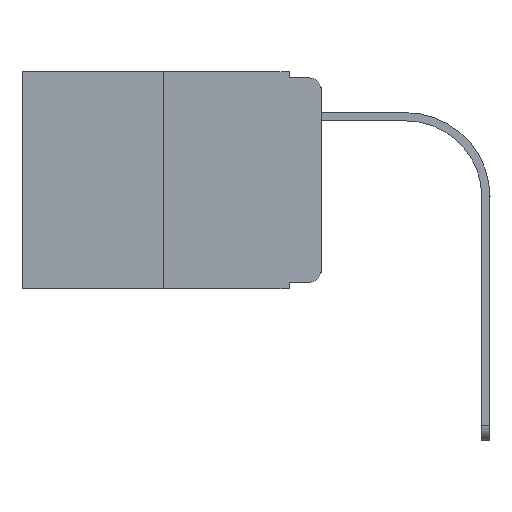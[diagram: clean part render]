
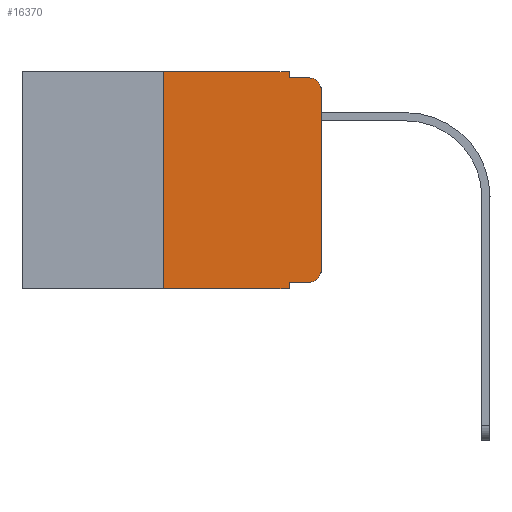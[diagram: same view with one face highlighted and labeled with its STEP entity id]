
A CAD part, left-side view. The second image highlights one B-rep face of the part: STEP entity #16370.
In plain terms, the highlighted planar face has unit normal (-1, 0, 0).
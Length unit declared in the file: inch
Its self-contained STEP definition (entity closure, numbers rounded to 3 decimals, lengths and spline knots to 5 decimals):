
#97 = DIRECTION ( 'NONE',  ( 0., -1., 0. ) ) ;
#289 = CARTESIAN_POINT ( 'NONE',  ( 0., 0.051, -0.333 ) ) ;
#323 = LINE ( 'NONE', #18625, #15803 ) ;
#576 = VERTEX_POINT ( 'NONE', #289 ) ;
#582 = DIRECTION ( 'NONE',  ( 0., 0., -1. ) ) ;
#863 = CARTESIAN_POINT ( 'NONE',  ( 0., 0., -0.03 ) ) ;
#1240 = ORIENTED_EDGE ( 'NONE', *, *, #13371, .F. ) ;
#1433 = EDGE_CURVE ( 'NONE', #3474, #18431, #18439, .T. ) ;
#1814 = CARTESIAN_POINT ( 'NONE',  ( 0., 0.473, 0. ) ) ;
#1886 = LINE ( 'NONE', #16724, #15252 ) ;
#2597 = LINE ( 'NONE', #4311, #8009 ) ;
#2624 = CARTESIAN_POINT ( 'NONE',  ( 0., 0.051, -0.01 ) ) ;
#2825 = VERTEX_POINT ( 'NONE', #2624 ) ;
#3166 = EDGE_CURVE ( 'NONE', #12573, #2825, #2597, .T. ) ;
#3474 = VERTEX_POINT ( 'NONE', #19797 ) ;
#3477 = CARTESIAN_POINT ( 'NONE',  ( 0., 0.25, -0.343 ) ) ;
#3517 = ORIENTED_EDGE ( 'NONE', *, *, #7996, .T. ) ;
#3905 = EDGE_CURVE ( 'NONE', #11225, #8612, #8434, .T. ) ;
#4311 = CARTESIAN_POINT ( 'NONE',  ( 0., 0.051, 0. ) ) ;
#4366 = EDGE_LOOP ( 'NONE', ( #14883, #16491, #10642, #6469, #14854, #1240, #18707, #10929, #3517, #11879 ) ) ;
#4749 = DIRECTION ( 'NONE',  ( 0., -1., 0. ) ) ;
#5303 = CARTESIAN_POINT ( 'NONE',  ( 0., 0.02, -0.313 ) ) ;
#6154 = LINE ( 'NONE', #9833, #7778 ) ;
#6469 = ORIENTED_EDGE ( 'NONE', *, *, #3166, .F. ) ;
#6566 = CARTESIAN_POINT ( 'NONE',  ( 0., 0.051, -0.01 ) ) ;
#6861 = CARTESIAN_POINT ( 'NONE',  ( 0., 0.473, 0. ) ) ;
#7022 = VECTOR ( 'NONE', #15597, 39.37008 ) ;
#7322 = CARTESIAN_POINT ( 'NONE',  ( 0., 0.02, -0.01 ) ) ;
#7508 = CARTESIAN_POINT ( 'NONE',  ( 0., 0.02, -0.03 ) ) ;
#7778 = VECTOR ( 'NONE', #7785, 39.37008 ) ;
#7785 = DIRECTION ( 'NONE',  ( 0., 0., 1. ) ) ;
#7996 = EDGE_CURVE ( 'NONE', #576, #3474, #323, .T. ) ;
#8009 = VECTOR ( 'NONE', #20795, 39.37008 ) ;
#8025 = EDGE_CURVE ( 'NONE', #576, #14619, #15379, .T. ) ;
#8121 = CARTESIAN_POINT ( 'NONE',  ( 0., 0., -0.313 ) ) ;
#8301 = EDGE_CURVE ( 'NONE', #2825, #8612, #12855, .T. ) ;
#8434 = CIRCLE ( 'NONE', #11191, 0.02 ) ;
#8502 = DIRECTION ( 'NONE',  ( 0., 0., 1. ) ) ;
#8612 = VERTEX_POINT ( 'NONE', #7322 ) ;
#8644 = LINE ( 'NONE', #1814, #15898 ) ;
#8743 = AXIS2_PLACEMENT_3D ( 'NONE', #5303, #11904, #13977 ) ;
#9833 = CARTESIAN_POINT ( 'NONE',  ( 0., 0., 0. ) ) ;
#10022 = DIRECTION ( 'NONE',  ( 0., 0., -1. ) ) ;
#10642 = ORIENTED_EDGE ( 'NONE', *, *, #8301, .F. ) ;
#10929 = ORIENTED_EDGE ( 'NONE', *, *, #8025, .F. ) ;
#11191 = AXIS2_PLACEMENT_3D ( 'NONE', #7508, #14213, #582 ) ;
#11225 = VERTEX_POINT ( 'NONE', #863 ) ;
#11263 = EDGE_CURVE ( 'NONE', #18431, #11225, #6154, .T. ) ;
#11444 = EDGE_CURVE ( 'NONE', #20512, #12573, #8644, .T. ) ;
#11551 = DIRECTION ( 'NONE',  ( 0., -1., 0. ) ) ;
#11879 = ORIENTED_EDGE ( 'NONE', *, *, #1433, .T. ) ;
#11904 = DIRECTION ( 'NONE',  ( -1., 0., 0. ) ) ;
#12204 = CARTESIAN_POINT ( 'NONE',  ( 0., 0.051, 0. ) ) ;
#12573 = VERTEX_POINT ( 'NONE', #18316 ) ;
#12811 = VECTOR ( 'NONE', #97, 39.37008 ) ;
#12855 = LINE ( 'NONE', #6566, #20891 ) ;
#12869 = CARTESIAN_POINT ( 'NONE',  ( 0., 0.473, -0.343 ) ) ;
#13191 = LINE ( 'NONE', #12869, #12811 ) ;
#13249 = PLANE ( 'NONE',  #19296 ) ;
#13371 = EDGE_CURVE ( 'NONE', #18485, #20512, #1886, .T. ) ;
#13977 = DIRECTION ( 'NONE',  ( 0., 0., -1. ) ) ;
#14129 = EDGE_CURVE ( 'NONE', #18485, #14619, #13191, .T. ) ;
#14213 = DIRECTION ( 'NONE',  ( -1., 0., 0. ) ) ;
#14619 = VERTEX_POINT ( 'NONE', #17947 ) ;
#14854 = ORIENTED_EDGE ( 'NONE', *, *, #11444, .F. ) ;
#14883 = ORIENTED_EDGE ( 'NONE', *, *, #11263, .T. ) ;
#14906 = FACE_OUTER_BOUND ( 'NONE', #4366, .T. ) ;
#15232 = DIRECTION ( 'NONE',  ( 1., 0., 0. ) ) ;
#15252 = VECTOR ( 'NONE', #8502, 39.37008 ) ;
#15379 = LINE ( 'NONE', #12204, #7022 ) ;
#15597 = DIRECTION ( 'NONE',  ( 0., 0., -1. ) ) ;
#15803 = VECTOR ( 'NONE', #18515, 39.37008 ) ;
#15898 = VECTOR ( 'NONE', #11551, 39.37008 ) ;
#16370 = ADVANCED_FACE ( 'NONE', ( #14906 ), #13249, .F. ) ;
#16491 = ORIENTED_EDGE ( 'NONE', *, *, #3905, .T. ) ;
#16724 = CARTESIAN_POINT ( 'NONE',  ( 0., 0.25, 0. ) ) ;
#17947 = CARTESIAN_POINT ( 'NONE',  ( 0., 0.051, -0.343 ) ) ;
#18316 = CARTESIAN_POINT ( 'NONE',  ( 0., 0.051, 0. ) ) ;
#18431 = VERTEX_POINT ( 'NONE', #8121 ) ;
#18439 = CIRCLE ( 'NONE', #8743, 0.02 ) ;
#18485 = VERTEX_POINT ( 'NONE', #3477 ) ;
#18515 = DIRECTION ( 'NONE',  ( 0., -1., 0. ) ) ;
#18625 = CARTESIAN_POINT ( 'NONE',  ( 0., 0.051, -0.333 ) ) ;
#18707 = ORIENTED_EDGE ( 'NONE', *, *, #14129, .T. ) ;
#19143 = CARTESIAN_POINT ( 'NONE',  ( 0., 0.25, 0. ) ) ;
#19296 = AXIS2_PLACEMENT_3D ( 'NONE', #6861, #15232, #10022 ) ;
#19797 = CARTESIAN_POINT ( 'NONE',  ( 0., 0.02, -0.333 ) ) ;
#20512 = VERTEX_POINT ( 'NONE', #19143 ) ;
#20795 = DIRECTION ( 'NONE',  ( 0., 0., -1. ) ) ;
#20891 = VECTOR ( 'NONE', #4749, 39.37008 ) ;
